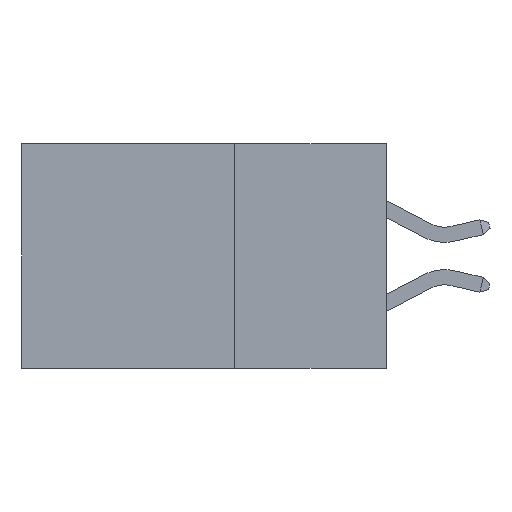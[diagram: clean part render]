
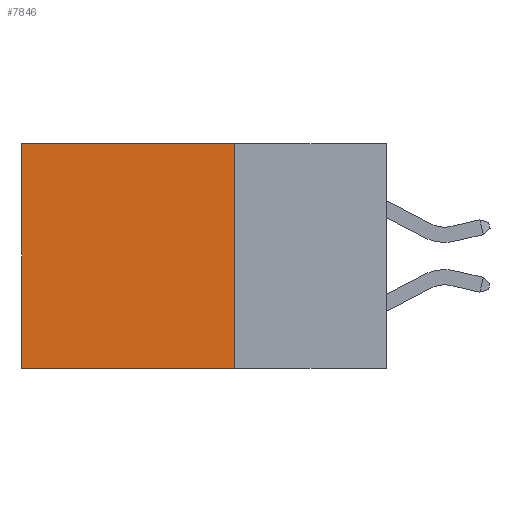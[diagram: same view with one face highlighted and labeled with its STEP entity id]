
A CAD part, left-side view. The second image highlights one B-rep face of the part: STEP entity #7846.
In plain terms, the highlighted planar face has unit normal (-1, 0, 0).
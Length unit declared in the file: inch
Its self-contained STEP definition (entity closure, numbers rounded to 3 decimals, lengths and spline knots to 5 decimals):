
#213 = AXIS2_PLACEMENT_3D ( 'NONE', #22949, #8299, #25398 ) ;
#1326 = DIRECTION ( 'NONE',  ( 0., 0., -1. ) ) ;
#1339 = FACE_OUTER_BOUND ( 'NONE', #12282, .T. ) ;
#1592 = CARTESIAN_POINT ( 'NONE',  ( 0.298, 0.25, 0. ) ) ;
#2938 = CARTESIAN_POINT ( 'NONE',  ( 0.298, 0.6, -0.37 ) ) ;
#3428 = CARTESIAN_POINT ( 'NONE',  ( 0.298, 0.25, -0.37 ) ) ;
#3433 = VERTEX_POINT ( 'NONE', #14794 ) ;
#4168 = LINE ( 'NONE', #15968, #29383 ) ;
#4963 = ORIENTED_EDGE ( 'NONE', *, *, #29322, .T. ) ;
#5842 = PLANE ( 'NONE',  #213 ) ;
#6488 = DIRECTION ( 'NONE',  ( 0., 1., 0. ) ) ;
#6803 = CARTESIAN_POINT ( 'NONE',  ( 0.298, 0.6, 0. ) ) ;
#7846 = ADVANCED_FACE ( 'NONE', ( #1339 ), #5842, .F. ) ;
#8299 = DIRECTION ( 'NONE',  ( 1., 0., 0. ) ) ;
#10325 = LINE ( 'NONE', #3428, #24089 ) ;
#10687 = DIRECTION ( 'NONE',  ( 0., 1., 0. ) ) ;
#11377 = CARTESIAN_POINT ( 'NONE',  ( 0.298, 0.6, 0. ) ) ;
#11564 = LINE ( 'NONE', #6803, #18098 ) ;
#12282 = EDGE_LOOP ( 'NONE', ( #4963, #26663, #21122, #15216 ) ) ;
#14101 = DIRECTION ( 'NONE',  ( 0., 0., -1. ) ) ;
#14794 = CARTESIAN_POINT ( 'NONE',  ( 0.298, 0.25, 0. ) ) ;
#15216 = ORIENTED_EDGE ( 'NONE', *, *, #29241, .T. ) ;
#15968 = CARTESIAN_POINT ( 'NONE',  ( 0.298, 0.25, 0. ) ) ;
#17011 = EDGE_CURVE ( 'NONE', #22130, #19661, #10325, .T. ) ;
#18098 = VECTOR ( 'NONE', #14101, 39.37008 ) ;
#19661 = VERTEX_POINT ( 'NONE', #2938 ) ;
#20413 = VECTOR ( 'NONE', #6488, 39.37008 ) ;
#20734 = CARTESIAN_POINT ( 'NONE',  ( 0.298, 0.25, -0.37 ) ) ;
#21122 = ORIENTED_EDGE ( 'NONE', *, *, #27407, .F. ) ;
#22130 = VERTEX_POINT ( 'NONE', #20734 ) ;
#22949 = CARTESIAN_POINT ( 'NONE',  ( 0.298, 0.25, 0. ) ) ;
#24089 = VECTOR ( 'NONE', #10687, 39.37008 ) ;
#25398 = DIRECTION ( 'NONE',  ( 0., 0., -1. ) ) ;
#26663 = ORIENTED_EDGE ( 'NONE', *, *, #17011, .F. ) ;
#26844 = LINE ( 'NONE', #1592, #20413 ) ;
#27407 = EDGE_CURVE ( 'NONE', #3433, #22130, #4168, .T. ) ;
#29241 = EDGE_CURVE ( 'NONE', #3433, #29931, #26844, .T. ) ;
#29322 = EDGE_CURVE ( 'NONE', #29931, #19661, #11564, .T. ) ;
#29383 = VECTOR ( 'NONE', #1326, 39.37008 ) ;
#29931 = VERTEX_POINT ( 'NONE', #11377 ) ;
